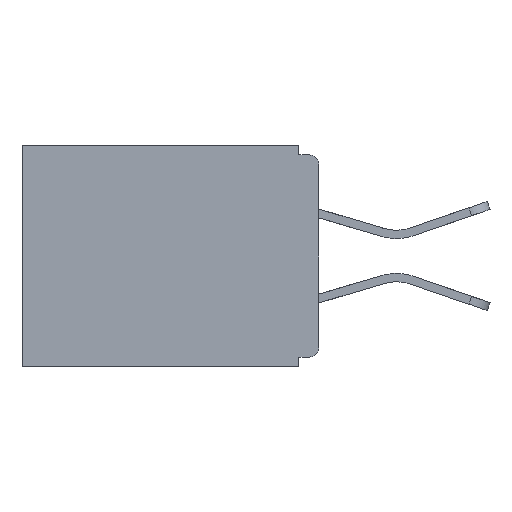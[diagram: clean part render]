
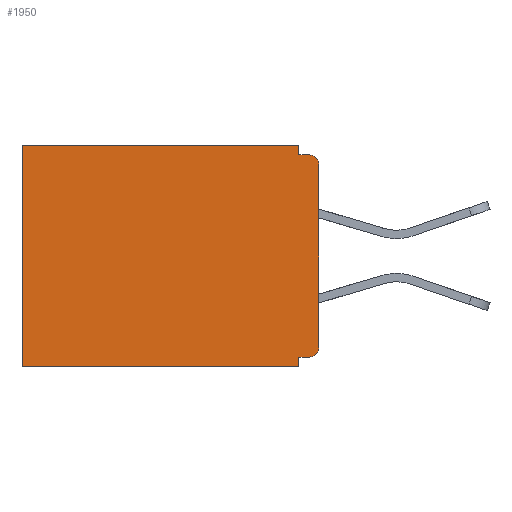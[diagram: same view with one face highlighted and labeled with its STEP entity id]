
A CAD part, left-side view. The second image highlights one B-rep face of the part: STEP entity #1950.
In plain terms, the highlighted planar face has unit normal (-1, 0, 0).
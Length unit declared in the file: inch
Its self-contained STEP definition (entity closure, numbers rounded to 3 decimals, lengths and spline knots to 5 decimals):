
#16 = ORIENTED_EDGE ( 'NONE', *, *, #2524, .F. ) ;
#97 = FACE_OUTER_BOUND ( 'NONE', #10405, .T. ) ;
#281 = ORIENTED_EDGE ( 'NONE', *, *, #8084, .T. ) ;
#496 = CIRCLE ( 'NONE', #3470, 0.015 ) ;
#722 = ORIENTED_EDGE ( 'NONE', *, *, #12151, .T. ) ;
#787 = VECTOR ( 'NONE', #7042, 39.37008 ) ;
#990 = EDGE_CURVE ( 'NONE', #11822, #8234, #1338, .T. ) ;
#1056 = VERTEX_POINT ( 'NONE', #22074 ) ;
#1338 = LINE ( 'NONE', #2497, #18613 ) ;
#1349 = CARTESIAN_POINT ( 'NONE',  ( 0.298, 0.46, 0. ) ) ;
#1703 = ORIENTED_EDGE ( 'NONE', *, *, #3284, .F. ) ;
#1841 = VECTOR ( 'NONE', #18533, 39.37008 ) ;
#1950 = ADVANCED_FACE ( 'NONE', ( #97 ), #11597, .F. ) ;
#2497 = CARTESIAN_POINT ( 'NONE',  ( 0.298, 0., 0. ) ) ;
#2524 = EDGE_CURVE ( 'NONE', #15810, #6352, #17356, .T. ) ;
#2689 = CARTESIAN_POINT ( 'NONE',  ( 0.298, 0.015, -0.313 ) ) ;
#3222 = CARTESIAN_POINT ( 'NONE',  ( 0.298, 0., -0.015 ) ) ;
#3284 = EDGE_CURVE ( 'NONE', #4112, #24297, #16381, .T. ) ;
#3437 = VECTOR ( 'NONE', #7036, 39.37008 ) ;
#3470 = AXIS2_PLACEMENT_3D ( 'NONE', #2689, #16011, #4610 ) ;
#3812 = ORIENTED_EDGE ( 'NONE', *, *, #15184, .F. ) ;
#4112 = VERTEX_POINT ( 'NONE', #14151 ) ;
#4610 = DIRECTION ( 'NONE',  ( 0., 0., -1. ) ) ;
#5167 = DIRECTION ( 'NONE',  ( 0., 0., -1. ) ) ;
#6352 = VERTEX_POINT ( 'NONE', #14433 ) ;
#6389 = DIRECTION ( 'NONE',  ( 0., 1., 0. ) ) ;
#6423 = EDGE_CURVE ( 'NONE', #24297, #15810, #7607, .T. ) ;
#6857 = LINE ( 'NONE', #22304, #1841 ) ;
#7036 = DIRECTION ( 'NONE',  ( 0., -1., 0. ) ) ;
#7042 = DIRECTION ( 'NONE',  ( 0., 0., -1. ) ) ;
#7184 = VECTOR ( 'NONE', #6389, 39.37008 ) ;
#7473 = ORIENTED_EDGE ( 'NONE', *, *, #990, .F. ) ;
#7607 = LINE ( 'NONE', #20234, #787 ) ;
#8084 = EDGE_CURVE ( 'NONE', #11822, #17546, #18765, .T. ) ;
#8234 = VERTEX_POINT ( 'NONE', #20167 ) ;
#8891 = AXIS2_PLACEMENT_3D ( 'NONE', #13749, #23132, #15669 ) ;
#8987 = AXIS2_PLACEMENT_3D ( 'NONE', #11899, #23284, #21282 ) ;
#9167 = DIRECTION ( 'NONE',  ( 0., 1., 0. ) ) ;
#9653 = CARTESIAN_POINT ( 'NONE',  ( 0.298, 0.031, -0.343 ) ) ;
#10008 = CARTESIAN_POINT ( 'NONE',  ( 0.298, 0.031, -0.015 ) ) ;
#10042 = VECTOR ( 'NONE', #5167, 39.37008 ) ;
#10043 = EDGE_CURVE ( 'NONE', #4112, #8234, #496, .T. ) ;
#10153 = DIRECTION ( 'NONE',  ( 0., 0., -1. ) ) ;
#10405 = EDGE_LOOP ( 'NONE', ( #281, #17656, #3812, #722, #12102, #16, #15375, #1703, #21276, #7473 ) ) ;
#11597 = PLANE ( 'NONE',  #8891 ) ;
#11822 = VERTEX_POINT ( 'NONE', #15695 ) ;
#11899 = CARTESIAN_POINT ( 'NONE',  ( 0.298, 0.015, -0.03 ) ) ;
#11954 = DIRECTION ( 'NONE',  ( 0., 0., -1. ) ) ;
#12031 = LINE ( 'NONE', #3222, #3437 ) ;
#12102 = ORIENTED_EDGE ( 'NONE', *, *, #22492, .T. ) ;
#12151 = EDGE_CURVE ( 'NONE', #23042, #1056, #6857, .T. ) ;
#12629 = CARTESIAN_POINT ( 'NONE',  ( 0.298, 0.015, -0.015 ) ) ;
#13749 = CARTESIAN_POINT ( 'NONE',  ( 0.298, 0., 0. ) ) ;
#13860 = VERTEX_POINT ( 'NONE', #10008 ) ;
#14151 = CARTESIAN_POINT ( 'NONE',  ( 0.298, 0.015, -0.328 ) ) ;
#14433 = CARTESIAN_POINT ( 'NONE',  ( 0.298, 0.46, -0.343 ) ) ;
#15184 = EDGE_CURVE ( 'NONE', #23042, #13860, #21299, .T. ) ;
#15375 = ORIENTED_EDGE ( 'NONE', *, *, #6423, .F. ) ;
#15472 = CARTESIAN_POINT ( 'NONE',  ( 0.298, 0., -0.343 ) ) ;
#15669 = DIRECTION ( 'NONE',  ( 0., 0., -1. ) ) ;
#15695 = CARTESIAN_POINT ( 'NONE',  ( 0.298, 0., -0.03 ) ) ;
#15810 = VERTEX_POINT ( 'NONE', #9653 ) ;
#16011 = DIRECTION ( 'NONE',  ( -1., 0., 0. ) ) ;
#16381 = LINE ( 'NONE', #18524, #24162 ) ;
#17110 = VECTOR ( 'NONE', #10153, 39.37008 ) ;
#17356 = LINE ( 'NONE', #15472, #7184 ) ;
#17546 = VERTEX_POINT ( 'NONE', #12629 ) ;
#17656 = ORIENTED_EDGE ( 'NONE', *, *, #23963, .F. ) ;
#18524 = CARTESIAN_POINT ( 'NONE',  ( 0.298, 0., -0.328 ) ) ;
#18533 = DIRECTION ( 'NONE',  ( 0., 1., 0. ) ) ;
#18613 = VECTOR ( 'NONE', #11954, 39.37008 ) ;
#18765 = CIRCLE ( 'NONE', #8987, 0.015 ) ;
#20167 = CARTESIAN_POINT ( 'NONE',  ( 0.298, 0., -0.313 ) ) ;
#20234 = CARTESIAN_POINT ( 'NONE',  ( 0.298, 0.031, -0.343 ) ) ;
#21073 = LINE ( 'NONE', #1349, #10042 ) ;
#21276 = ORIENTED_EDGE ( 'NONE', *, *, #10043, .T. ) ;
#21282 = DIRECTION ( 'NONE',  ( 0., 0., -1. ) ) ;
#21299 = LINE ( 'NONE', #23367, #17110 ) ;
#21528 = CARTESIAN_POINT ( 'NONE',  ( 0.298, 0.031, -0.328 ) ) ;
#22074 = CARTESIAN_POINT ( 'NONE',  ( 0.298, 0.46, 0. ) ) ;
#22304 = CARTESIAN_POINT ( 'NONE',  ( 0.298, 0., 0. ) ) ;
#22492 = EDGE_CURVE ( 'NONE', #1056, #6352, #21073, .T. ) ;
#22835 = CARTESIAN_POINT ( 'NONE',  ( 0.298, 0.031, 0. ) ) ;
#23042 = VERTEX_POINT ( 'NONE', #22835 ) ;
#23132 = DIRECTION ( 'NONE',  ( 1., 0., 0. ) ) ;
#23284 = DIRECTION ( 'NONE',  ( -1., 0., 0. ) ) ;
#23367 = CARTESIAN_POINT ( 'NONE',  ( 0.298, 0.031, -0.343 ) ) ;
#23963 = EDGE_CURVE ( 'NONE', #13860, #17546, #12031, .T. ) ;
#24162 = VECTOR ( 'NONE', #9167, 39.37008 ) ;
#24297 = VERTEX_POINT ( 'NONE', #21528 ) ;
